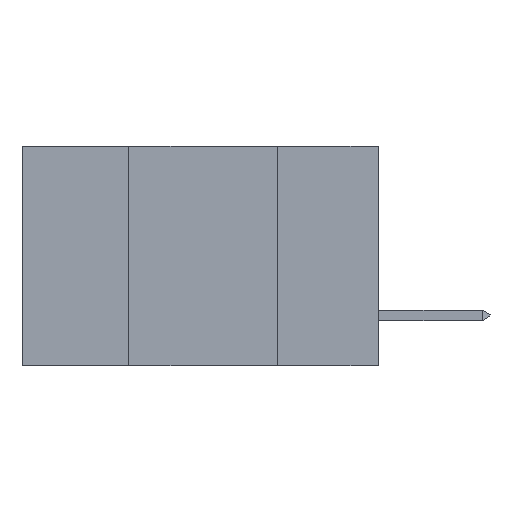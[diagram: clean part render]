
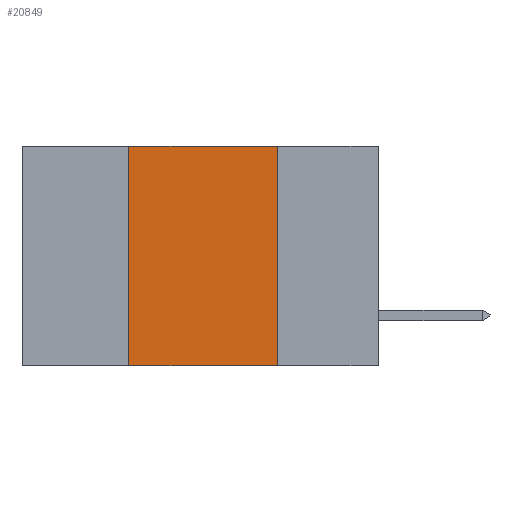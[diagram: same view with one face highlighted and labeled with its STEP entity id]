
A CAD part, left-side view. The second image highlights one B-rep face of the part: STEP entity #20849.
In plain terms, the highlighted planar face has unit normal (-1, 0, 0).
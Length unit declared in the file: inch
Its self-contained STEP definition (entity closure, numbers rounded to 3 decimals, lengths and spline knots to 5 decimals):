
#1225 = EDGE_CURVE ( 'NONE', #20917, #7742, #10675, .T. ) ;
#1392 = ORIENTED_EDGE ( 'NONE', *, *, #1225, .F. ) ;
#1410 = CARTESIAN_POINT ( 'NONE',  ( 0., 0.6, 0. ) ) ;
#2756 = DIRECTION ( 'NONE',  ( 0., -1., 0. ) ) ;
#4771 = VERTEX_POINT ( 'NONE', #21839 ) ;
#4897 = PLANE ( 'NONE',  #20421 ) ;
#6664 = EDGE_CURVE ( 'NONE', #7742, #4771, #26839, .T. ) ;
#6914 = VECTOR ( 'NONE', #8192, 39.37008 ) ;
#7199 = CARTESIAN_POINT ( 'NONE',  ( 0., 0.6, 0. ) ) ;
#7742 = VERTEX_POINT ( 'NONE', #17760 ) ;
#7817 = VERTEX_POINT ( 'NONE', #17374 ) ;
#8192 = DIRECTION ( 'NONE',  ( 0., -1., 0. ) ) ;
#8530 = DIRECTION ( 'NONE',  ( 0., 0., -1. ) ) ;
#9129 = EDGE_LOOP ( 'NONE', ( #20380, #13735, #1392, #21684 ) ) ;
#9983 = CARTESIAN_POINT ( 'NONE',  ( 0., 0.42, -0.37 ) ) ;
#10658 = CARTESIAN_POINT ( 'NONE',  ( 0., 0.6, -0.37 ) ) ;
#10675 = LINE ( 'NONE', #21633, #11398 ) ;
#10746 = EDGE_CURVE ( 'NONE', #4771, #7817, #29171, .T. ) ;
#11331 = EDGE_CURVE ( 'NONE', #20917, #7817, #17866, .T. ) ;
#11398 = VECTOR ( 'NONE', #22112, 39.37008 ) ;
#13735 = ORIENTED_EDGE ( 'NONE', *, *, #6664, .F. ) ;
#14415 = DIRECTION ( 'NONE',  ( 0., 0., -1. ) ) ;
#15483 = CARTESIAN_POINT ( 'NONE',  ( 0., 0.17, 0. ) ) ;
#17374 = CARTESIAN_POINT ( 'NONE',  ( 0., 0.17, -0.37 ) ) ;
#17760 = CARTESIAN_POINT ( 'NONE',  ( 0., 0.42, 0. ) ) ;
#17866 = LINE ( 'NONE', #10658, #6914 ) ;
#19900 = VECTOR ( 'NONE', #2756, 39.37008 ) ;
#20380 = ORIENTED_EDGE ( 'NONE', *, *, #10746, .F. ) ;
#20421 = AXIS2_PLACEMENT_3D ( 'NONE', #7199, #28277, #14415 ) ;
#20849 = ADVANCED_FACE ( 'NONE', ( #29525 ), #4897, .F. ) ;
#20917 = VERTEX_POINT ( 'NONE', #9983 ) ;
#21633 = CARTESIAN_POINT ( 'NONE',  ( 0., 0.42, 0. ) ) ;
#21684 = ORIENTED_EDGE ( 'NONE', *, *, #11331, .T. ) ;
#21839 = CARTESIAN_POINT ( 'NONE',  ( 0., 0.17, 0. ) ) ;
#22112 = DIRECTION ( 'NONE',  ( 0., 0., 1. ) ) ;
#22292 = VECTOR ( 'NONE', #8530, 39.37008 ) ;
#26839 = LINE ( 'NONE', #1410, #19900 ) ;
#28277 = DIRECTION ( 'NONE',  ( 1., 0., 0. ) ) ;
#29171 = LINE ( 'NONE', #15483, #22292 ) ;
#29525 = FACE_OUTER_BOUND ( 'NONE', #9129, .T. ) ;
